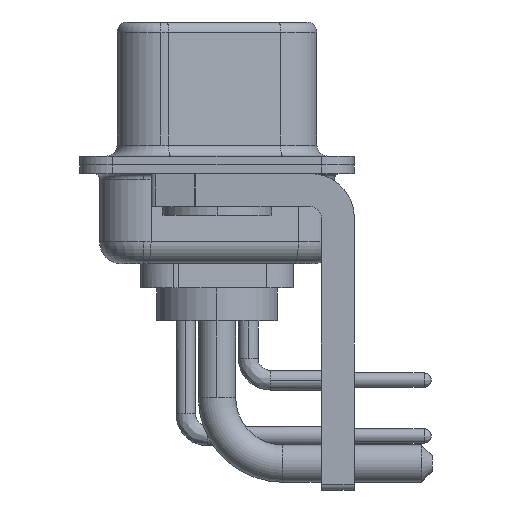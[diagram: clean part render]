
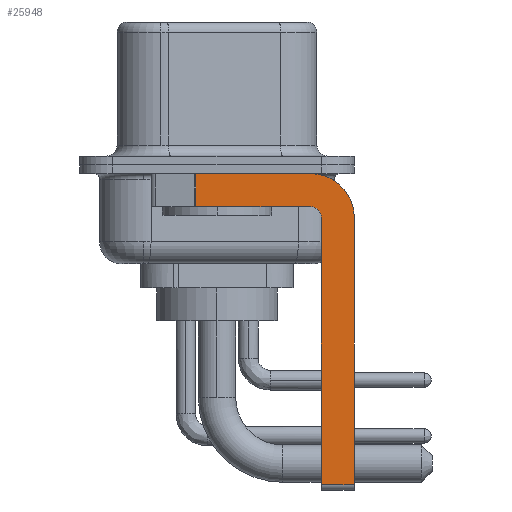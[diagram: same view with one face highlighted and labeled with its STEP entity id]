
A CAD part, left-side view. The second image highlights one B-rep face of the part: STEP entity #25948.
In plain terms, the highlighted planar face has unit normal (-1, 0, 0).
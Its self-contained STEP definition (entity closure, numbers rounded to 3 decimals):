
#163 = CARTESIAN_POINT ( 'NONE',  ( -2.9, -6.25, -14.55 ) ) ;
#412 = CARTESIAN_POINT ( 'NONE',  ( -2.9, -6.25, -2.4 ) ) ;
#548 = EDGE_CURVE ( 'NONE', #18828, #13586, #16635, .T. ) ;
#865 = CARTESIAN_POINT ( 'NONE',  ( -2.9, -4.75, -14.8 ) ) ;
#941 = CARTESIAN_POINT ( 'NONE',  ( -2.9, -4.25, -14.55 ) ) ;
#1083 = VECTOR ( 'NONE', #18787, 1000. ) ;
#1116 = CARTESIAN_POINT ( 'NONE',  ( -2.9, 0.978, -0.4 ) ) ;
#1128 = EDGE_CURVE ( 'NONE', #1263, #21158, #20400, .T. ) ;
#1263 = VERTEX_POINT ( 'NONE', #21480 ) ;
#1677 = FACE_OUTER_BOUND ( 'NONE', #14349, .T. ) ;
#2363 = DIRECTION ( 'NONE',  ( 0., 0., -1. ) ) ;
#2786 = ORIENTED_EDGE ( 'NONE', *, *, #1128, .F. ) ;
#3481 = VECTOR ( 'NONE', #22143, 1000. ) ;
#3734 = VECTOR ( 'NONE', #18720, 1000. ) ;
#4990 = DIRECTION ( 'NONE',  ( 0., 0., 1. ) ) ;
#5689 = DIRECTION ( 'NONE',  ( 0., 0., -1. ) ) ;
#6088 = EDGE_CURVE ( 'NONE', #18828, #1263, #17940, .T. ) ;
#7132 = ORIENTED_EDGE ( 'NONE', *, *, #548, .T. ) ;
#7423 = CARTESIAN_POINT ( 'NONE',  ( -2.9, 0.978, -1.9 ) ) ;
#8838 = VERTEX_POINT ( 'NONE', #19522 ) ;
#9477 = DIRECTION ( 'NONE',  ( 1., 0., 0. ) ) ;
#9819 = ORIENTED_EDGE ( 'NONE', *, *, #16058, .F. ) ;
#9973 = VECTOR ( 'NONE', #12044, 1000. ) ;
#10589 = CARTESIAN_POINT ( 'NONE',  ( -2.9, -4.25, -1.9 ) ) ;
#10682 = AXIS2_PLACEMENT_3D ( 'NONE', #29092, #24627, #19734 ) ;
#11229 = EDGE_CURVE ( 'NONE', #21158, #26547, #12526, .T. ) ;
#11672 = DIRECTION ( 'NONE',  ( -1., 0., 0. ) ) ;
#12044 = DIRECTION ( 'NONE',  ( 0., 0., -1. ) ) ;
#12210 = LINE ( 'NONE', #941, #3734 ) ;
#12458 = ORIENTED_EDGE ( 'NONE', *, *, #16029, .F. ) ;
#12526 = LINE ( 'NONE', #23778, #13757 ) ;
#13124 = LINE ( 'NONE', #10589, #3481 ) ;
#13586 = VERTEX_POINT ( 'NONE', #15544 ) ;
#13757 = VECTOR ( 'NONE', #5689, 1000. ) ;
#13971 = CARTESIAN_POINT ( 'NONE',  ( -2.9, -4.25, -2.4 ) ) ;
#14349 = EDGE_LOOP ( 'NONE', ( #25985, #7132, #29131, #12458, #9819, #15942, #19894, #2786 ) ) ;
#15544 = CARTESIAN_POINT ( 'NONE',  ( -2.9, 0.978, -1.9 ) ) ;
#15942 = ORIENTED_EDGE ( 'NONE', *, *, #28516, .T. ) ;
#16029 = EDGE_CURVE ( 'NONE', #20983, #26469, #21868, .T. ) ;
#16058 = EDGE_CURVE ( 'NONE', #8838, #20983, #16566, .T. ) ;
#16566 = LINE ( 'NONE', #865, #1083 ) ;
#16635 = LINE ( 'NONE', #7423, #9973 ) ;
#17153 = EDGE_CURVE ( 'NONE', #26469, #13586, #13124, .T. ) ;
#17641 = CARTESIAN_POINT ( 'NONE',  ( -2.9, 3., -0.4 ) ) ;
#17940 = LINE ( 'NONE', #17641, #19159 ) ;
#18720 = DIRECTION ( 'NONE',  ( 0., -1., 0. ) ) ;
#18787 = DIRECTION ( 'NONE',  ( 0., 0., 1. ) ) ;
#18828 = VERTEX_POINT ( 'NONE', #1116 ) ;
#18923 = CARTESIAN_POINT ( 'NONE',  ( -2.9, -4.25, -2.4 ) ) ;
#19159 = VECTOR ( 'NONE', #20168, 1000. ) ;
#19522 = CARTESIAN_POINT ( 'NONE',  ( -2.9, -4.75, -14.55 ) ) ;
#19734 = DIRECTION ( 'NONE',  ( 0., 0., -1. ) ) ;
#19894 = ORIENTED_EDGE ( 'NONE', *, *, #11229, .F. ) ;
#20168 = DIRECTION ( 'NONE',  ( 0., -1., 0. ) ) ;
#20400 = CIRCLE ( 'NONE', #25628, 2. ) ;
#20983 = VERTEX_POINT ( 'NONE', #22321 ) ;
#21158 = VERTEX_POINT ( 'NONE', #412 ) ;
#21480 = CARTESIAN_POINT ( 'NONE',  ( -2.9, -4.25, -0.4 ) ) ;
#21868 = CIRCLE ( 'NONE', #22331, 0.5 ) ;
#22143 = DIRECTION ( 'NONE',  ( 0., 1., 0. ) ) ;
#22321 = CARTESIAN_POINT ( 'NONE',  ( -2.9, -4.75, -2.4 ) ) ;
#22331 = AXIS2_PLACEMENT_3D ( 'NONE', #18923, #11672, #4990 ) ;
#23778 = CARTESIAN_POINT ( 'NONE',  ( -2.9, -6.25, -2.4 ) ) ;
#24455 = CARTESIAN_POINT ( 'NONE',  ( -2.9, -4.25, -1.9 ) ) ;
#24627 = DIRECTION ( 'NONE',  ( 1., 0., 0. ) ) ;
#25628 = AXIS2_PLACEMENT_3D ( 'NONE', #13971, #9477, #2363 ) ;
#25948 = ADVANCED_FACE ( 'NONE', ( #1677 ), #26567, .F. ) ;
#25985 = ORIENTED_EDGE ( 'NONE', *, *, #6088, .F. ) ;
#26469 = VERTEX_POINT ( 'NONE', #24455 ) ;
#26547 = VERTEX_POINT ( 'NONE', #163 ) ;
#26567 = PLANE ( 'NONE',  #10682 ) ;
#28516 = EDGE_CURVE ( 'NONE', #8838, #26547, #12210, .T. ) ;
#29092 = CARTESIAN_POINT ( 'NONE',  ( -2.9, -4.25, -2.4 ) ) ;
#29131 = ORIENTED_EDGE ( 'NONE', *, *, #17153, .F. ) ;
